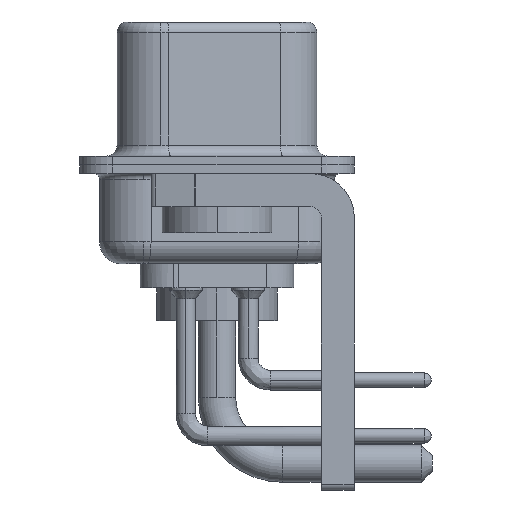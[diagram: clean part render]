
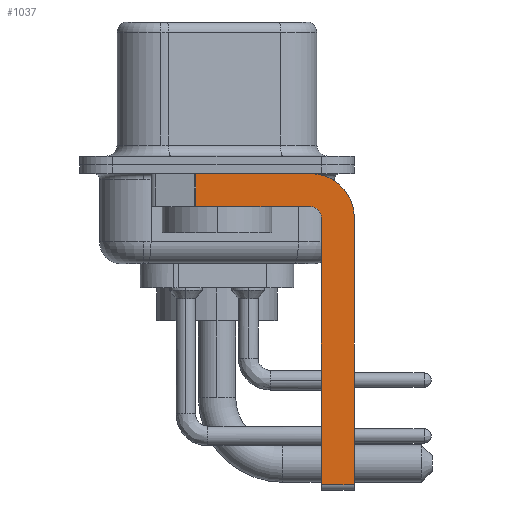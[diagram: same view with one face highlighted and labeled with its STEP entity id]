
A CAD part, left-side view. The second image highlights one B-rep face of the part: STEP entity #1037.
In plain terms, the highlighted planar face has unit normal (-1, 0, 0).
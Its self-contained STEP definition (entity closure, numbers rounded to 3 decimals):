
#34 = VERTEX_POINT ( 'NONE', #15514 ) ;
#762 = LINE ( 'NONE', #3939, #21316 ) ;
#820 = AXIS2_PLACEMENT_3D ( 'NONE', #8257, #11893, #2707 ) ;
#921 = AXIS2_PLACEMENT_3D ( 'NONE', #15556, #19448, #3302 ) ;
#1037 = ADVANCED_FACE ( 'NONE', ( #20323 ), #13569, .F. ) ;
#1320 = CARTESIAN_POINT ( 'NONE',  ( -2.9, -6.25, -14.55 ) ) ;
#1451 = DIRECTION ( 'NONE',  ( 0., 0., -1. ) ) ;
#1696 = EDGE_CURVE ( 'NONE', #6865, #17101, #2669, .T. ) ;
#1831 = CARTESIAN_POINT ( 'NONE',  ( -2.9, -6.25, -2.4 ) ) ;
#2669 = CIRCLE ( 'NONE', #20723, 2. ) ;
#2675 = DIRECTION ( 'NONE',  ( 0., -1., 0. ) ) ;
#2707 = DIRECTION ( 'NONE',  ( 0., 0., -1. ) ) ;
#3233 = EDGE_CURVE ( 'NONE', #14625, #19430, #18939, .T. ) ;
#3302 = DIRECTION ( 'NONE',  ( 0., 0., 1. ) ) ;
#3546 = ORIENTED_EDGE ( 'NONE', *, *, #16249, .F. ) ;
#3683 = LINE ( 'NONE', #12648, #8615 ) ;
#3804 = DIRECTION ( 'NONE',  ( 0., 0., 1. ) ) ;
#3939 = CARTESIAN_POINT ( 'NONE',  ( -2.9, -4.25, -1.9 ) ) ;
#4163 = CARTESIAN_POINT ( 'NONE',  ( -2.9, -4.75, -14.8 ) ) ;
#4319 = CARTESIAN_POINT ( 'NONE',  ( -2.9, -4.25, -0.4 ) ) ;
#5395 = ORIENTED_EDGE ( 'NONE', *, *, #12014, .F. ) ;
#5544 = ORIENTED_EDGE ( 'NONE', *, *, #6888, .F. ) ;
#6071 = DIRECTION ( 'NONE',  ( 0., 1., 0. ) ) ;
#6166 = DIRECTION ( 'NONE',  ( 0., 0., -1. ) ) ;
#6865 = VERTEX_POINT ( 'NONE', #4319 ) ;
#6888 = EDGE_CURVE ( 'NONE', #8745, #6865, #7986, .T. ) ;
#7308 = EDGE_CURVE ( 'NONE', #17327, #34, #762, .T. ) ;
#7986 = LINE ( 'NONE', #22337, #16809 ) ;
#8257 = CARTESIAN_POINT ( 'NONE',  ( -2.9, -4.25, -2.4 ) ) ;
#8615 = VECTOR ( 'NONE', #1451, 1000. ) ;
#8745 = VERTEX_POINT ( 'NONE', #11644 ) ;
#9210 = VECTOR ( 'NONE', #3804, 1000. ) ;
#9927 = ORIENTED_EDGE ( 'NONE', *, *, #12305, .F. ) ;
#9984 = CARTESIAN_POINT ( 'NONE',  ( -2.9, -4.25, -14.55 ) ) ;
#10910 = ORIENTED_EDGE ( 'NONE', *, *, #11623, .T. ) ;
#10911 = EDGE_LOOP ( 'NONE', ( #5544, #10910, #13934, #9927, #5395, #21907, #3546, #21869 ) ) ;
#11385 = CARTESIAN_POINT ( 'NONE',  ( -2.9, -4.25, -1.9 ) ) ;
#11566 = CARTESIAN_POINT ( 'NONE',  ( -2.9, -4.75, -14.55 ) ) ;
#11623 = EDGE_CURVE ( 'NONE', #8745, #34, #17248, .T. ) ;
#11644 = CARTESIAN_POINT ( 'NONE',  ( -2.9, 0.978, -0.4 ) ) ;
#11893 = DIRECTION ( 'NONE',  ( 1., 0., 0. ) ) ;
#12014 = EDGE_CURVE ( 'NONE', #14625, #17689, #20306, .T. ) ;
#12305 = EDGE_CURVE ( 'NONE', #17689, #17327, #16411, .T. ) ;
#12648 = CARTESIAN_POINT ( 'NONE',  ( -2.9, -6.25, -2.4 ) ) ;
#12817 = DIRECTION ( 'NONE',  ( 1., 0., 0. ) ) ;
#13569 = PLANE ( 'NONE',  #820 ) ;
#13934 = ORIENTED_EDGE ( 'NONE', *, *, #7308, .F. ) ;
#14473 = VECTOR ( 'NONE', #18839, 1000. ) ;
#14625 = VERTEX_POINT ( 'NONE', #11566 ) ;
#15039 = CARTESIAN_POINT ( 'NONE',  ( -2.9, -4.25, -2.4 ) ) ;
#15514 = CARTESIAN_POINT ( 'NONE',  ( -2.9, 0.978, -1.9 ) ) ;
#15556 = CARTESIAN_POINT ( 'NONE',  ( -2.9, -4.25, -2.4 ) ) ;
#16249 = EDGE_CURVE ( 'NONE', #17101, #19430, #3683, .T. ) ;
#16411 = CIRCLE ( 'NONE', #921, 0.5 ) ;
#16584 = DIRECTION ( 'NONE',  ( 0., 0., -1. ) ) ;
#16809 = VECTOR ( 'NONE', #2675, 1000. ) ;
#17101 = VERTEX_POINT ( 'NONE', #1831 ) ;
#17248 = LINE ( 'NONE', #20553, #20169 ) ;
#17327 = VERTEX_POINT ( 'NONE', #11385 ) ;
#17689 = VERTEX_POINT ( 'NONE', #21832 ) ;
#18839 = DIRECTION ( 'NONE',  ( 0., -1., 0. ) ) ;
#18939 = LINE ( 'NONE', #9984, #14473 ) ;
#19430 = VERTEX_POINT ( 'NONE', #1320 ) ;
#19448 = DIRECTION ( 'NONE',  ( -1., 0., 0. ) ) ;
#20169 = VECTOR ( 'NONE', #6166, 1000. ) ;
#20306 = LINE ( 'NONE', #4163, #9210 ) ;
#20323 = FACE_OUTER_BOUND ( 'NONE', #10911, .T. ) ;
#20553 = CARTESIAN_POINT ( 'NONE',  ( -2.9, 0.978, -1.9 ) ) ;
#20723 = AXIS2_PLACEMENT_3D ( 'NONE', #15039, #12817, #16584 ) ;
#21316 = VECTOR ( 'NONE', #6071, 1000. ) ;
#21832 = CARTESIAN_POINT ( 'NONE',  ( -2.9, -4.75, -2.4 ) ) ;
#21869 = ORIENTED_EDGE ( 'NONE', *, *, #1696, .F. ) ;
#21907 = ORIENTED_EDGE ( 'NONE', *, *, #3233, .T. ) ;
#22337 = CARTESIAN_POINT ( 'NONE',  ( -2.9, 3., -0.4 ) ) ;
